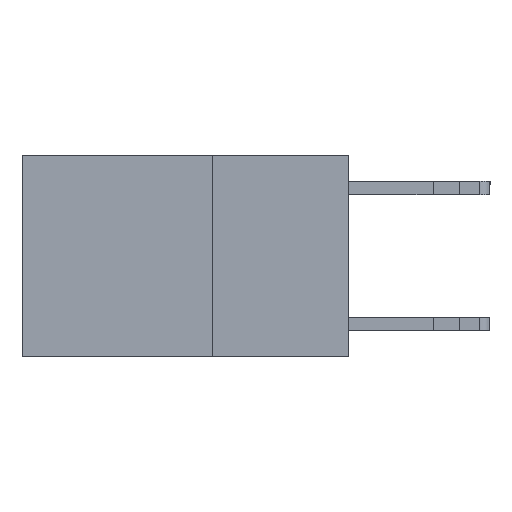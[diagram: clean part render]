
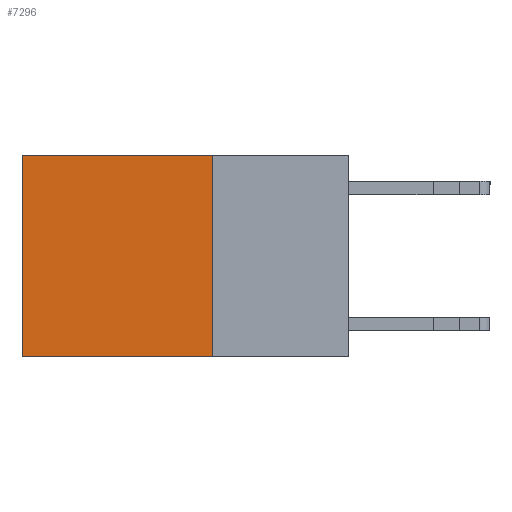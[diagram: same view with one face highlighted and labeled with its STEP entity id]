
A CAD part, left-side view. The second image highlights one B-rep face of the part: STEP entity #7296.
In plain terms, the highlighted planar face has unit normal (-1, 0, 0).
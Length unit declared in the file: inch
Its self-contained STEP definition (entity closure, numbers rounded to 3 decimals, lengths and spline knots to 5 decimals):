
#862 = CARTESIAN_POINT ( 'NONE',  ( 0.2625, 0.25, 0. ) ) ;
#864 = CARTESIAN_POINT ( 'NONE',  ( 0.2625, 0.25, -0.37 ) ) ;
#1272 = ORIENTED_EDGE ( 'NONE', *, *, #18580, .T. ) ;
#2389 = VERTEX_POINT ( 'NONE', #6265 ) ;
#2958 = ORIENTED_EDGE ( 'NONE', *, *, #18212, .F. ) ;
#3272 = LINE ( 'NONE', #6703, #18097 ) ;
#3487 = CARTESIAN_POINT ( 'NONE',  ( 0.2625, 0.6, 0. ) ) ;
#4371 = PLANE ( 'NONE',  #17170 ) ;
#4784 = VECTOR ( 'NONE', #6510, 39.37008 ) ;
#5163 = VECTOR ( 'NONE', #9411, 39.37008 ) ;
#5563 = ORIENTED_EDGE ( 'NONE', *, *, #19187, .F. ) ;
#6265 = CARTESIAN_POINT ( 'NONE',  ( 0.2625, 0.25, 0. ) ) ;
#6510 = DIRECTION ( 'NONE',  ( 0., 0., -1. ) ) ;
#6554 = EDGE_CURVE ( 'NONE', #11921, #9966, #9686, .T. ) ;
#6703 = CARTESIAN_POINT ( 'NONE',  ( 0.2625, 0.25, 0. ) ) ;
#6794 = ORIENTED_EDGE ( 'NONE', *, *, #6554, .T. ) ;
#7296 = ADVANCED_FACE ( 'NONE', ( #19369 ), #4371, .F. ) ;
#8048 = CARTESIAN_POINT ( 'NONE',  ( 0.2625, 0.6, 0. ) ) ;
#9096 = LINE ( 'NONE', #862, #5163 ) ;
#9411 = DIRECTION ( 'NONE',  ( 0., 1., 0. ) ) ;
#9686 = LINE ( 'NONE', #8048, #4784 ) ;
#9966 = VERTEX_POINT ( 'NONE', #15582 ) ;
#11059 = CARTESIAN_POINT ( 'NONE',  ( 0.2625, 0.25, 0. ) ) ;
#11464 = CARTESIAN_POINT ( 'NONE',  ( 0.2625, 0.25, -0.37 ) ) ;
#11921 = VERTEX_POINT ( 'NONE', #3487 ) ;
#13046 = DIRECTION ( 'NONE',  ( 0., 0., -1. ) ) ;
#13930 = DIRECTION ( 'NONE',  ( 0., 0., -1. ) ) ;
#15582 = CARTESIAN_POINT ( 'NONE',  ( 0.2625, 0.6, -0.37 ) ) ;
#16331 = VECTOR ( 'NONE', #19557, 39.37008 ) ;
#17170 = AXIS2_PLACEMENT_3D ( 'NONE', #11059, #17742, #13930 ) ;
#17742 = DIRECTION ( 'NONE',  ( 1., 0., 0. ) ) ;
#18097 = VECTOR ( 'NONE', #13046, 39.37008 ) ;
#18212 = EDGE_CURVE ( 'NONE', #2389, #20026, #3272, .T. ) ;
#18580 = EDGE_CURVE ( 'NONE', #2389, #11921, #9096, .T. ) ;
#19187 = EDGE_CURVE ( 'NONE', #20026, #9966, #21314, .T. ) ;
#19369 = FACE_OUTER_BOUND ( 'NONE', #20066, .T. ) ;
#19557 = DIRECTION ( 'NONE',  ( 0., 1., 0. ) ) ;
#20026 = VERTEX_POINT ( 'NONE', #864 ) ;
#20066 = EDGE_LOOP ( 'NONE', ( #6794, #5563, #2958, #1272 ) ) ;
#21314 = LINE ( 'NONE', #11464, #16331 ) ;
